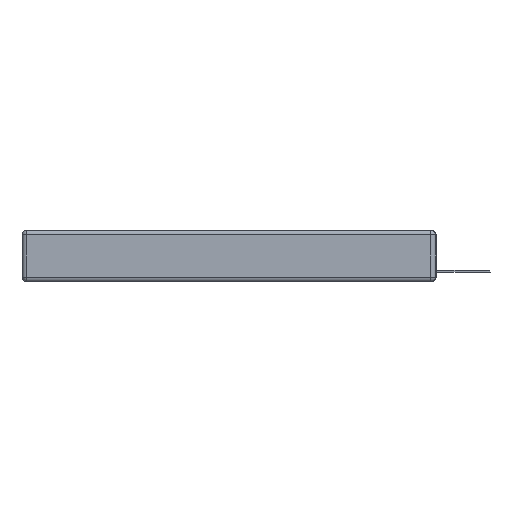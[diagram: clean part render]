
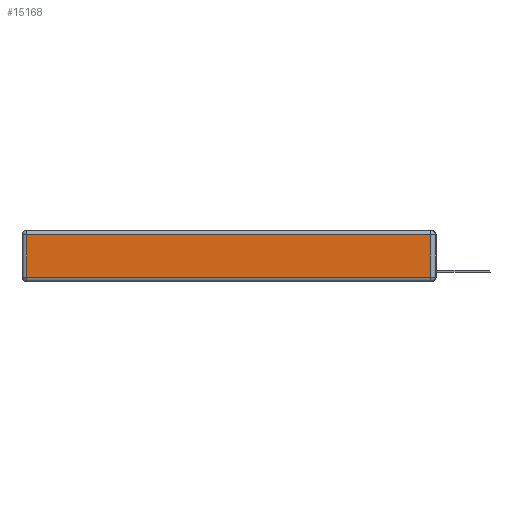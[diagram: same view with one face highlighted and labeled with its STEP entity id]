
A CAD part, left-side view. The second image highlights one B-rep face of the part: STEP entity #15168.
In plain terms, the highlighted planar face has unit normal (-1, 0, 0).
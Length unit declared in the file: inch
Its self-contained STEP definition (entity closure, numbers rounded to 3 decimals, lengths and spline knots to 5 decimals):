
#615 = EDGE_CURVE ( 'NONE', #21897, #3726, #9167, .T. ) ;
#725 = CARTESIAN_POINT ( 'NONE',  ( 0., 2.72, -0.343 ) ) ;
#933 = CARTESIAN_POINT ( 'NONE',  ( 0., 0.03, -0.343 ) ) ;
#1147 = DIRECTION ( 'NONE',  ( 0., 1., 0. ) ) ;
#1237 = CARTESIAN_POINT ( 'NONE',  ( 0., 0., -0.343 ) ) ;
#1301 = VERTEX_POINT ( 'NONE', #9173 ) ;
#1840 = ORIENTED_EDGE ( 'NONE', *, *, #17800, .T. ) ;
#2277 = EDGE_CURVE ( 'NONE', #21277, #21897, #8148, .T. ) ;
#2502 = ORIENTED_EDGE ( 'NONE', *, *, #23019, .T. ) ;
#3726 = VERTEX_POINT ( 'NONE', #13205 ) ;
#3765 = AXIS2_PLACEMENT_3D ( 'NONE', #1237, #16534, #14593 ) ;
#6358 = DIRECTION ( 'NONE',  ( 0., -1., 0. ) ) ;
#7785 = EDGE_LOOP ( 'NONE', ( #19090, #1840, #2502, #24191 ) ) ;
#8148 = LINE ( 'NONE', #725, #16479 ) ;
#9167 = LINE ( 'NONE', #17752, #20522 ) ;
#9173 = CARTESIAN_POINT ( 'NONE',  ( 0., 0.03, -0.03 ) ) ;
#10701 = CARTESIAN_POINT ( 'NONE',  ( 0., 2.75, -0.03 ) ) ;
#11202 = VECTOR ( 'NONE', #12202, 39.37008 ) ;
#12202 = DIRECTION ( 'NONE',  ( 0., 0., 1. ) ) ;
#12383 = LINE ( 'NONE', #933, #11202 ) ;
#12647 = DIRECTION ( 'NONE',  ( 0., 0., -1. ) ) ;
#13205 = CARTESIAN_POINT ( 'NONE',  ( 0., 0.03, -0.313 ) ) ;
#14067 = VECTOR ( 'NONE', #1147, 39.37008 ) ;
#14593 = DIRECTION ( 'NONE',  ( 0., 0., 1. ) ) ;
#15168 = ADVANCED_FACE ( 'NONE', ( #19391 ), #24159, .T. ) ;
#16479 = VECTOR ( 'NONE', #12647, 39.37008 ) ;
#16534 = DIRECTION ( 'NONE',  ( -1., 0., 0. ) ) ;
#17752 = CARTESIAN_POINT ( 'NONE',  ( 0., 0., -0.313 ) ) ;
#17800 = EDGE_CURVE ( 'NONE', #3726, #1301, #12383, .T. ) ;
#19090 = ORIENTED_EDGE ( 'NONE', *, *, #615, .T. ) ;
#19391 = FACE_OUTER_BOUND ( 'NONE', #7785, .T. ) ;
#20405 = CARTESIAN_POINT ( 'NONE',  ( 0., 2.72, -0.03 ) ) ;
#20522 = VECTOR ( 'NONE', #6358, 39.37008 ) ;
#20958 = LINE ( 'NONE', #10701, #14067 ) ;
#21277 = VERTEX_POINT ( 'NONE', #20405 ) ;
#21897 = VERTEX_POINT ( 'NONE', #24066 ) ;
#23019 = EDGE_CURVE ( 'NONE', #1301, #21277, #20958, .T. ) ;
#24066 = CARTESIAN_POINT ( 'NONE',  ( 0., 2.72, -0.313 ) ) ;
#24159 = PLANE ( 'NONE',  #3765 ) ;
#24191 = ORIENTED_EDGE ( 'NONE', *, *, #2277, .T. ) ;
